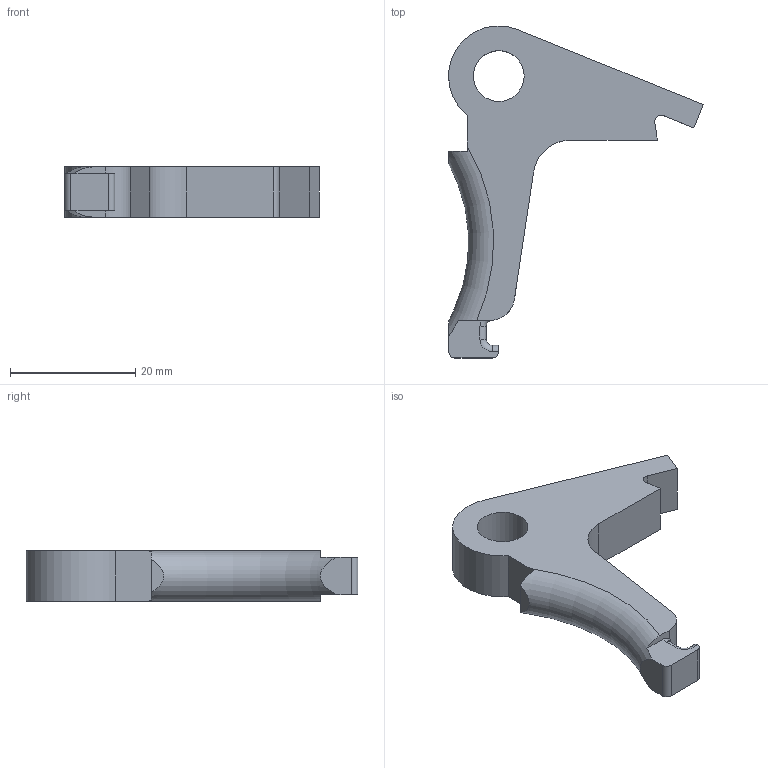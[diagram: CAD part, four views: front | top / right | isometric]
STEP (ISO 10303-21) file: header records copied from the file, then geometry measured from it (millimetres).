
FILE_DESCRIPTION((''),'2;1');
FILE_NAME('PM422Trigger2.stp','2015-08-22T19:04:22',('JamesRPatrick'),(''),'Autodesk Inventor 2012','Autodesk Inventor 2012','');
FILE_SCHEMA(('AUTOMOTIVE_DESIGN { 1 0 10303 214 1 1 1 1 }'));
Length unit declared in the file: millimetre
Products named in the file (1): PM422Trigger2
Bounding box: 40.67 x 52.99 x 8 mm (x, y, z)
Volume: 5899.6 mm3; surface area: 3011.6 mm2
Topology: 1 solids, 1 shells, 38 faces, 102 edges, 66 vertices
Faces by surface type: plane 20, cylinder 13, torus 5
Full cylindrical faces by diameter (mm): 8.1 x1
Entity records: 1295 total; most frequent: CARTESIAN_POINT 312, ORIENTED_EDGE 202, DIRECTION 199, EDGE_CURVE 101, AXIS2_PLACEMENT_3D 73, VERTEX_POINT 66, VECTOR 53, LINE 53
